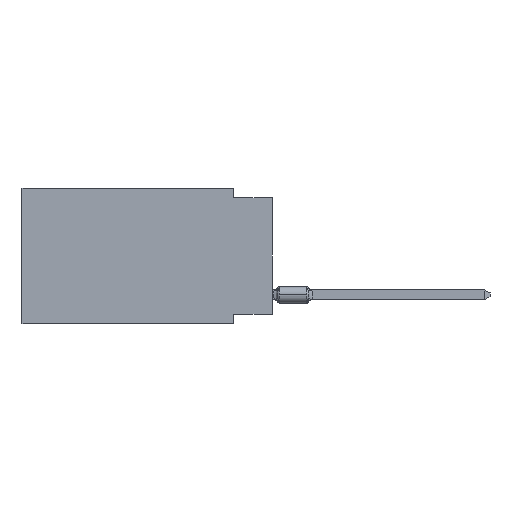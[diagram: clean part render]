
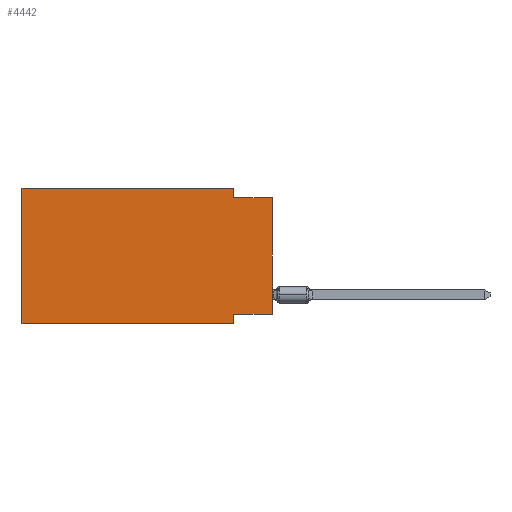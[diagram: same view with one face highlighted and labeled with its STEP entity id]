
A CAD part, left-side view. The second image highlights one B-rep face of the part: STEP entity #4442.
In plain terms, the highlighted planar face has unit normal (-1, 0, 0).
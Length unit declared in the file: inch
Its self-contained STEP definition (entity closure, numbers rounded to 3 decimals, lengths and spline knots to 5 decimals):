
#284 = DIRECTION ( 'NONE',  ( 1., 0., 0. ) ) ;
#1460 = DIRECTION ( 'NONE',  ( 0., 0., -1. ) ) ;
#2055 = LINE ( 'NONE', #11000, #4031 ) ;
#2476 = DIRECTION ( 'NONE',  ( 0., 0., -1. ) ) ;
#2552 = DIRECTION ( 'NONE',  ( 0., 1., 0. ) ) ;
#3058 = LINE ( 'NONE', #7159, #26133 ) ;
#3146 = LINE ( 'NONE', #12072, #4344 ) ;
#3275 = EDGE_LOOP ( 'NONE', ( #28415, #12674, #28756, #19619, #16958, #10730, #14526, #4929 ) ) ;
#4031 = VECTOR ( 'NONE', #28129, 39.37008 ) ;
#4303 = CARTESIAN_POINT ( 'NONE',  ( 0., 0., 0. ) ) ;
#4344 = VECTOR ( 'NONE', #2552, 39.37008 ) ;
#4385 = CARTESIAN_POINT ( 'NONE',  ( 0., 0.645, 0. ) ) ;
#4442 = ADVANCED_FACE ( 'NONE', ( #6463 ), #24587, .F. ) ;
#4635 = CARTESIAN_POINT ( 'NONE',  ( 0., 0.1, -0.35 ) ) ;
#4929 = ORIENTED_EDGE ( 'NONE', *, *, #20049, .F. ) ;
#6463 = FACE_OUTER_BOUND ( 'NONE', #3275, .T. ) ;
#6639 = EDGE_CURVE ( 'NONE', #7742, #10425, #24354, .T. ) ;
#6860 = VECTOR ( 'NONE', #19087, 39.37008 ) ;
#7116 = CARTESIAN_POINT ( 'NONE',  ( 0., 0.645, 0. ) ) ;
#7159 = CARTESIAN_POINT ( 'NONE',  ( 0., 0.645, -0.35 ) ) ;
#7742 = VERTEX_POINT ( 'NONE', #12652 ) ;
#7767 = LINE ( 'NONE', #12292, #26377 ) ;
#8240 = VERTEX_POINT ( 'NONE', #28695 ) ;
#8384 = EDGE_CURVE ( 'NONE', #15253, #21922, #7767, .T. ) ;
#10172 = CARTESIAN_POINT ( 'NONE',  ( 0., 0.645, 0. ) ) ;
#10425 = VERTEX_POINT ( 'NONE', #28093 ) ;
#10705 = CARTESIAN_POINT ( 'NONE',  ( 0., 0.1, -0.025 ) ) ;
#10730 = ORIENTED_EDGE ( 'NONE', *, *, #19258, .T. ) ;
#10922 = DIRECTION ( 'NONE',  ( 0., 0., 1. ) ) ;
#11000 = CARTESIAN_POINT ( 'NONE',  ( 0., 0.1, -0.35 ) ) ;
#11355 = LINE ( 'NONE', #7116, #26005 ) ;
#11845 = EDGE_CURVE ( 'NONE', #8240, #18296, #2055, .T. ) ;
#12072 = CARTESIAN_POINT ( 'NONE',  ( 0., 0., -0.325 ) ) ;
#12225 = LINE ( 'NONE', #27728, #21321 ) ;
#12292 = CARTESIAN_POINT ( 'NONE',  ( 0., 0.1, 0. ) ) ;
#12452 = EDGE_CURVE ( 'NONE', #17041, #15253, #26115, .T. ) ;
#12652 = CARTESIAN_POINT ( 'NONE',  ( 0., 0., -0.325 ) ) ;
#12674 = ORIENTED_EDGE ( 'NONE', *, *, #25444, .F. ) ;
#13351 = DIRECTION ( 'NONE',  ( 0., 0., 1. ) ) ;
#13874 = DIRECTION ( 'NONE',  ( 0., -1., 0. ) ) ;
#14526 = ORIENTED_EDGE ( 'NONE', *, *, #11845, .F. ) ;
#15015 = CARTESIAN_POINT ( 'NONE',  ( 0., 0.645, 0. ) ) ;
#15253 = VERTEX_POINT ( 'NONE', #24008 ) ;
#16958 = ORIENTED_EDGE ( 'NONE', *, *, #25330, .F. ) ;
#17041 = VERTEX_POINT ( 'NONE', #15015 ) ;
#18101 = AXIS2_PLACEMENT_3D ( 'NONE', #4385, #284, #2476 ) ;
#18296 = VERTEX_POINT ( 'NONE', #4635 ) ;
#19087 = DIRECTION ( 'NONE',  ( 0., -1., 0. ) ) ;
#19258 = EDGE_CURVE ( 'NONE', #27491, #18296, #3058, .T. ) ;
#19619 = ORIENTED_EDGE ( 'NONE', *, *, #12452, .F. ) ;
#20049 = EDGE_CURVE ( 'NONE', #7742, #8240, #3146, .T. ) ;
#20576 = DIRECTION ( 'NONE',  ( 0., -1., 0. ) ) ;
#21136 = VECTOR ( 'NONE', #13351, 39.37008 ) ;
#21321 = VECTOR ( 'NONE', #20576, 39.37008 ) ;
#21922 = VERTEX_POINT ( 'NONE', #10705 ) ;
#22975 = CARTESIAN_POINT ( 'NONE',  ( 0., 0.645, -0.35 ) ) ;
#24008 = CARTESIAN_POINT ( 'NONE',  ( 0., 0.1, 0. ) ) ;
#24354 = LINE ( 'NONE', #4303, #21136 ) ;
#24587 = PLANE ( 'NONE',  #18101 ) ;
#25330 = EDGE_CURVE ( 'NONE', #27491, #17041, #11355, .T. ) ;
#25444 = EDGE_CURVE ( 'NONE', #21922, #10425, #12225, .T. ) ;
#26005 = VECTOR ( 'NONE', #10922, 39.37008 ) ;
#26115 = LINE ( 'NONE', #10172, #6860 ) ;
#26133 = VECTOR ( 'NONE', #13874, 39.37008 ) ;
#26377 = VECTOR ( 'NONE', #1460, 39.37008 ) ;
#27491 = VERTEX_POINT ( 'NONE', #22975 ) ;
#27728 = CARTESIAN_POINT ( 'NONE',  ( 0., 0., -0.025 ) ) ;
#28093 = CARTESIAN_POINT ( 'NONE',  ( 0., 0., -0.025 ) ) ;
#28129 = DIRECTION ( 'NONE',  ( 0., 0., -1. ) ) ;
#28415 = ORIENTED_EDGE ( 'NONE', *, *, #6639, .T. ) ;
#28695 = CARTESIAN_POINT ( 'NONE',  ( 0., 0.1, -0.325 ) ) ;
#28756 = ORIENTED_EDGE ( 'NONE', *, *, #8384, .F. ) ;
